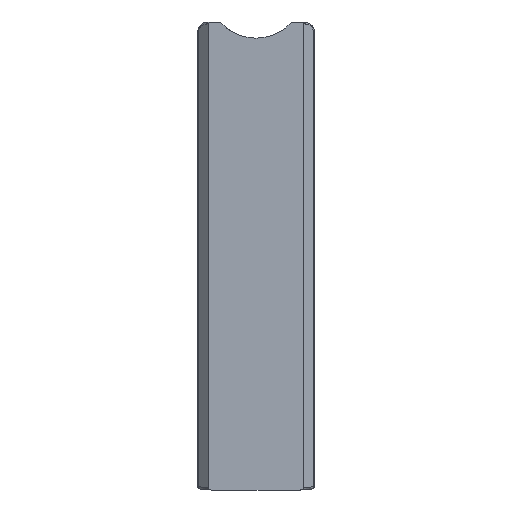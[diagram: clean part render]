
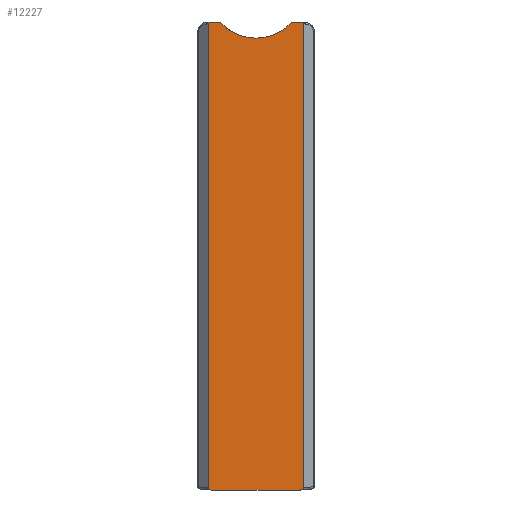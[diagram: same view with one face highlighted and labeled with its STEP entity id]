
A CAD part, front view. The second image highlights one B-rep face of the part: STEP entity #12227.
In plain terms, the highlighted planar face has unit normal (0, -1, 0).
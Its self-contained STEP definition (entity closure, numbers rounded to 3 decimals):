
#52=ELLIPSE('',#13145,0.567,0.4);
#53=ELLIPSE('',#13147,0.566,0.4);
#57=ELLIPSE('',#13166,0.567,0.4);
#61=ELLIPSE('',#13173,0.566,0.4);
#939=PLANE('',#13186);
#1781=FACE_OUTER_BOUND('',#2536,.T.);
#2536=EDGE_LOOP('',(#11317,#11318,#11319,#11320,#11321,#11322,#11323,#11324,
#11325,#11326,#11327,#11328));
#3570=LINE('',#26247,#4631);
#3584=LINE('',#26352,#4645);
#3607=LINE('',#26512,#4668);
#3608=LINE('',#26513,#4669);
#3609=LINE('',#26517,#4670);
#4631=VECTOR('',#15928,10.);
#4645=VECTOR('',#15984,10.);
#4668=VECTOR('',#16079,10.);
#4669=VECTOR('',#16080,10.);
#4670=VECTOR('',#16085,10.);
#5024=CIRCLE('',#13185,0.4);
#5025=CIRCLE('',#13187,9.);
#5026=CIRCLE('',#13188,0.4);
#6073=VERTEX_POINT('',#26244);
#6074=VERTEX_POINT('',#26246);
#6088=VERTEX_POINT('',#26337);
#6089=VERTEX_POINT('',#26341);
#6090=VERTEX_POINT('',#26342);
#6091=VERTEX_POINT('',#26351);
#6102=VERTEX_POINT('',#26434);
#6107=VERTEX_POINT('',#26450);
#6108=VERTEX_POINT('',#26451);
#6116=VERTEX_POINT('',#26506);
#6117=VERTEX_POINT('',#26507);
#6118=VERTEX_POINT('',#26514);
#7793=EDGE_CURVE('',#6074,#6073,#3570,.T.);
#7813=EDGE_CURVE('',#6074,#6088,#52,.T.);
#7815=EDGE_CURVE('',#6089,#6090,#53,.T.);
#7820=EDGE_CURVE('',#6090,#6091,#3584,.T.);
#7838=EDGE_CURVE('',#6102,#6073,#57,.T.);
#7846=EDGE_CURVE('',#6107,#6108,#61,.T.);
#7862=EDGE_CURVE('',#6116,#6117,#5024,.T.);
#7865=EDGE_CURVE('',#6102,#6108,#3607,.T.);
#7866=EDGE_CURVE('',#6117,#6107,#3608,.T.);
#7867=EDGE_CURVE('',#6116,#6118,#5025,.T.);
#7868=EDGE_CURVE('',#6091,#6118,#5026,.T.);
#7869=EDGE_CURVE('',#6088,#6089,#3609,.T.);
#11317=ORIENTED_EDGE('',*,*,#7813,.F.);
#11318=ORIENTED_EDGE('',*,*,#7793,.T.);
#11319=ORIENTED_EDGE('',*,*,#7838,.F.);
#11320=ORIENTED_EDGE('',*,*,#7865,.T.);
#11321=ORIENTED_EDGE('',*,*,#7846,.F.);
#11322=ORIENTED_EDGE('',*,*,#7866,.F.);
#11323=ORIENTED_EDGE('',*,*,#7862,.F.);
#11324=ORIENTED_EDGE('',*,*,#7867,.T.);
#11325=ORIENTED_EDGE('',*,*,#7868,.F.);
#11326=ORIENTED_EDGE('',*,*,#7820,.F.);
#11327=ORIENTED_EDGE('',*,*,#7815,.F.);
#11328=ORIENTED_EDGE('',*,*,#7869,.F.);
#12227=ADVANCED_FACE('',(#1781),#939,.T.);
#13145=AXIS2_PLACEMENT_3D('',#26338,#15967,#15968);
#13147=AXIS2_PLACEMENT_3D('',#26343,#15972,#15973);
#13166=AXIS2_PLACEMENT_3D('',#26435,#16021,#16022);
#13173=AXIS2_PLACEMENT_3D('',#26452,#16039,#16040);
#13185=AXIS2_PLACEMENT_3D('',#26508,#16073,#16074);
#13186=AXIS2_PLACEMENT_3D('',#26511,#16077,#16078);
#13187=AXIS2_PLACEMENT_3D('',#26515,#16081,#16082);
#13188=AXIS2_PLACEMENT_3D('',#26516,#16083,#16084);
#15928=DIRECTION('',(1.,0.,0.));
#15967=DIRECTION('center_axis',(0.,1.,0.));
#15968=DIRECTION('ref_axis',(-0.996,0.,0.087));
#15972=DIRECTION('center_axis',(0.,1.,0.));
#15973=DIRECTION('ref_axis',(-1.,0.,0.));
#15984=DIRECTION('',(1.,0.,0.));
#16021=DIRECTION('center_axis',(0.,1.,0.));
#16022=DIRECTION('ref_axis',(0.996,0.,0.087));
#16039=DIRECTION('center_axis',(0.,1.,0.));
#16040=DIRECTION('ref_axis',(1.,0.,0.));
#16073=DIRECTION('center_axis',(0.,1.,0.));
#16074=DIRECTION('ref_axis',(-0.399,0.,0.917));
#16077=DIRECTION('center_axis',(0.,-1.,0.));
#16078=DIRECTION('ref_axis',(1.,0.,0.));
#16079=DIRECTION('',(0.,0.,1.));
#16080=DIRECTION('',(1.,0.,0.));
#16081=DIRECTION('center_axis',(0.,1.,0.));
#16082=DIRECTION('ref_axis',(1.,0.,0.));
#16083=DIRECTION('center_axis',(0.,1.,0.));
#16084=DIRECTION('ref_axis',(0.399,0.,0.917));
#16085=DIRECTION('',(0.,0.,1.));
#26244=CARTESIAN_POINT('',(19.155,0.,-50.));
#26246=CARTESIAN_POINT('',(2.645,0.,-50.));
#26247=CARTESIAN_POINT('',(2.045,0.,-50.));
#26337=CARTESIAN_POINT('',(2.045,0.,-49.574));
#26338=CARTESIAN_POINT('Origin',(2.61,0.,
-49.598));
#26341=CARTESIAN_POINT('',(2.045,0.,36.6));
#26342=CARTESIAN_POINT('',(2.61,0.,37.));
#26343=CARTESIAN_POINT('Origin',(2.61,0.,36.6));
#26351=CARTESIAN_POINT('',(4.015,0.,37.));
#26352=CARTESIAN_POINT('',(2.045,0.,37.));
#26434=CARTESIAN_POINT('',(19.755,0.,-49.574));
#26435=CARTESIAN_POINT('Origin',(19.19,0.,-49.598));
#26450=CARTESIAN_POINT('',(19.19,0.,37.));
#26451=CARTESIAN_POINT('',(19.755,0.,36.6));
#26452=CARTESIAN_POINT('Origin',(19.19,0.,36.6));
#26506=CARTESIAN_POINT('',(17.492,0.,36.872));
#26507=CARTESIAN_POINT('',(17.785,0.,37.));
#26508=CARTESIAN_POINT('Origin',(17.785,0.,
36.6));
#26511=CARTESIAN_POINT('Origin',(2.045,0.,
-50.));
#26512=CARTESIAN_POINT('',(19.755,0.,-50.));
#26513=CARTESIAN_POINT('',(2.045,0.,37.));
#26514=CARTESIAN_POINT('',(4.308,0.,36.872));
#26515=CARTESIAN_POINT('Origin',(10.9,0.,43.));
#26516=CARTESIAN_POINT('Origin',(4.015,0.,
36.6));
#26517=CARTESIAN_POINT('',(2.045,0.,-50.));
